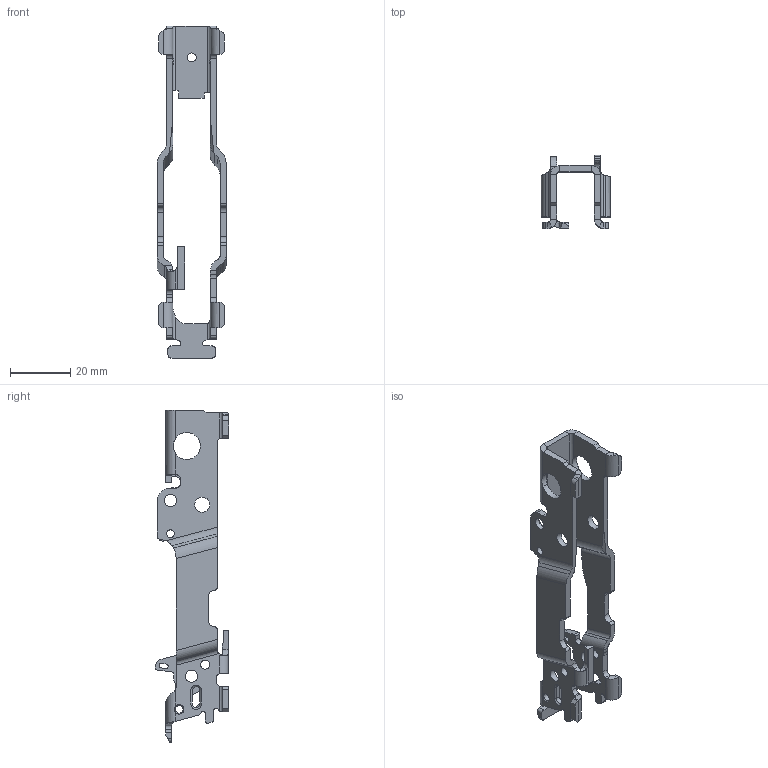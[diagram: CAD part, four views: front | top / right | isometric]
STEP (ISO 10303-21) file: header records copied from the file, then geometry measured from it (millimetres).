
FILE_DESCRIPTION(/* description */ (''),/* implementation_level */ '2;1');
FILE_NAME(/* name */ 'P320 FCU with Manual Safety Cutout.step',/* time_stamp */ '2024-01-17T21:57:13-05:00',/* author */ (''),/* organization */ (''),/* preprocessor_version */ 'ST-DEVELOPER v20',/* originating_system */ 'Autodesk Translation Framework v12.14.0.127',/* authorisation */ '');
FILE_SCHEMA (('AUTOMOTIVE_DESIGN { 1 0 10303 214 3 1 1 }'));
Length unit declared in the file: millimetre
Products named in the file (1): Test 320 Bent
Bounding box: 23.15 x 24.31 x 110.25 mm (x, y, z)
Volume: 6831.8 mm3; surface area: 8592.3 mm2
Topology: 1 solids, 1 shells, 322 faces, 890 edges, 564 vertices
Faces by surface type: plane 152, cylinder 146, bspline 16, cone 8
Full cylindrical faces by diameter (mm): 1.6 x2, 2.55 x4, 3 x1, 3.03 x2, 4 x3, 5 x2
Entity records: 10721 total; most frequent: CARTESIAN_POINT 2357, ORIENTED_EDGE 1780, DIRECTION 1718, EDGE_CURVE 890, AXIS2_PLACEMENT_3D 579, VERTEX_POINT 564, LINE 560, VECTOR 560
